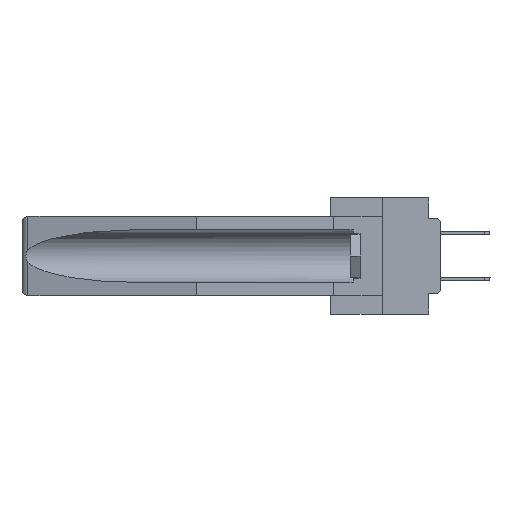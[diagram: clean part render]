
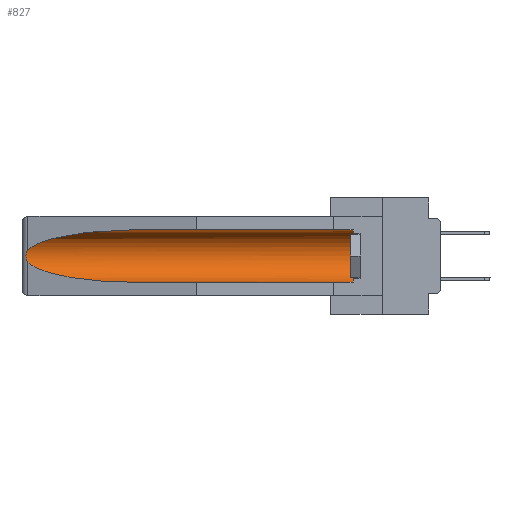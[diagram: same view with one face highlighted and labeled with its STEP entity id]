
A CAD part, left-side view. The second image highlights one B-rep face of the part: STEP entity #827.
In plain terms, the highlighted cylindrical face has radius 2.857 mm (diameter 5.715 mm), a partial arc.
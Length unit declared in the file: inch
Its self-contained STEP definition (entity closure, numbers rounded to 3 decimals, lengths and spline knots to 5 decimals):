
#441 = CARTESIAN_POINT ( 'NONE',  ( 0.2673, 1.5327, -0.16383 ) ) ;
#774 = CIRCLE ( 'NONE', #2671, 0.1125 ) ;
#827 = ADVANCED_FACE ( 'NONE', ( #22563 ), #9307, .F. ) ;
#1045 = CARTESIAN_POINT ( 'NONE',  ( 0.155, 1.07973, -0.059 ) ) ;
#1121 = CARTESIAN_POINT ( 'NONE',  ( 0.155, 1.07973, -0.284 ) ) ;
#1220 = CARTESIAN_POINT ( 'NONE',  ( 0.155, 1.07973, -0.059 ) ) ;
#1238 = ORIENTED_EDGE ( 'NONE', *, *, #25741, .T. ) ;
#1357 = CARTESIAN_POINT ( 'NONE',  ( 0.155, 0.126, -0.284 ) ) ;
#1448 = CARTESIAN_POINT ( 'NONE',  ( 0.26537, 1.52718, -0.14972 ) ) ;
#1894 = AXIS2_PLACEMENT_3D ( 'NONE', #6697, #4351, #22425 ) ;
#2671 = AXIS2_PLACEMENT_3D ( 'NONE', #27612, #11398, #7012 ) ;
#2932 = CARTESIAN_POINT ( 'NONE',  ( 0.2673, 1.53269, -0.17917 ) ) ;
#3207 = VERTEX_POINT ( 'NONE', #1121 ) ;
#4351 = DIRECTION ( 'NONE',  ( 0., 1., 0. ) ) ;
#5395 = CARTESIAN_POINT ( 'NONE',  ( 0.155, -0.30754, -0.059 ) ) ;
#6697 = CARTESIAN_POINT ( 'NONE',  ( 0.155, -0.30754, -0.1715 ) ) ;
#7012 = DIRECTION ( 'NONE',  ( 0., 0., 1. ) ) ;
#7700 = CARTESIAN_POINT ( 'NONE',  ( 0.25451, 1.48313, -0.24835 ) ) ;
#7730 = VERTEX_POINT ( 'NONE', #1357 ) ;
#8001 = CARTESIAN_POINT ( 'NONE',  ( 0.21114, 1.30732, -0.284 ) ) ;
#9307 = CYLINDRICAL_SURFACE ( 'NONE', #1894, 0.1125 ) ;
#9392 = CARTESIAN_POINT ( 'NONE',  ( 0.26597, 1.52961, -0.15275 ) ) ;
#10302 = CARTESIAN_POINT ( 'NONE',  ( 0.25451, 1.48313, -0.09465 ) ) ;
#11138 = VECTOR ( 'NONE', #12366, 39.37008 ) ;
#11343 = ORIENTED_EDGE ( 'NONE', *, *, #18758, .T. ) ;
#11398 = DIRECTION ( 'NONE',  ( 0., -1., 0. ) ) ;
#11415 = VERTEX_POINT ( 'NONE', #1448 ) ;
#11786 = CARTESIAN_POINT ( 'NONE',  ( 0.155, 0.126, -0.059 ) ) ;
#11888 = CARTESIAN_POINT ( 'NONE',  ( 0.26537, 1.52718, -0.19328 ) ) ;
#12366 = DIRECTION ( 'NONE',  ( 0., 1., 0. ) ) ;
#14098 = CARTESIAN_POINT ( 'NONE',  ( 0.26654, 1.53092, -0.15636 ) ) ;
#14947 = VECTOR ( 'NONE', #24578, 39.37008 ) ;
#15572 = ORIENTED_EDGE ( 'NONE', *, *, #17820, .T. ) ;
#16286 = CARTESIAN_POINT ( 'NONE',  ( 0.26537, 1.52718, -0.14972 ) ) ;
#16301 = ORIENTED_EDGE ( 'NONE', *, *, #27776, .T. ) ;
#16391 = EDGE_LOOP ( 'NONE', ( #11343, #16301, #1238, #21153, #17786, #15572 ) ) ;
#16468 = EDGE_CURVE ( 'NONE', #7730, #21875, #774, .T. ) ;
#16647 = CARTESIAN_POINT ( 'NONE',  ( 0.155, 1.07973, -0.284 ) ) ;
#17065 = CARTESIAN_POINT ( 'NONE',  ( 0.26537, 1.52718, -0.14972 ) ) ;
#17400 = EDGE_CURVE ( 'NONE', #7730, #3207, #20894, .T. ) ;
#17786 = ORIENTED_EDGE ( 'NONE', *, *, #16468, .T. ) ;
#17820 = EDGE_CURVE ( 'NONE', #21875, #26985, #26948, .T. ) ;
#18070 = CARTESIAN_POINT ( 'NONE',  ( 0.2675, 1.53308, -0.16763 ) ) ;
#18363 = CARTESIAN_POINT ( 'NONE',  ( 0.2675, 1.53308, -0.17534 ) ) ;
#18758 = EDGE_CURVE ( 'NONE', #26985, #11415, #19409, .T. ) ;
#19409 =( BOUNDED_CURVE ( )  B_SPLINE_CURVE ( 3, ( #1045, #21054, #10302, #17065 ),
 .UNSPECIFIED., .F., .F. ) 
 B_SPLINE_CURVE_WITH_KNOTS ( ( 4, 4 ),
 ( 4.71239, 6.08839 ),
 .UNSPECIFIED. ) 
 CURVE ( )  GEOMETRIC_REPRESENTATION_ITEM ( )  RATIONAL_B_SPLINE_CURVE ( ( 1., 0.848, 0.848, 1. ) ) 
 REPRESENTATION_ITEM ( '' )  );
#19684 = CARTESIAN_POINT ( 'NONE',  ( 0.26537, 1.52718, -0.19328 ) ) ;
#20894 = LINE ( 'NONE', #21046, #11138 ) ;
#21046 = CARTESIAN_POINT ( 'NONE',  ( 0.155, -0.30754, -0.284 ) ) ;
#21054 = CARTESIAN_POINT ( 'NONE',  ( 0.21114, 1.30732, -0.059 ) ) ;
#21153 = ORIENTED_EDGE ( 'NONE', *, *, #17400, .F. ) ;
#21875 = VERTEX_POINT ( 'NONE', #11786 ) ;
#22425 = DIRECTION ( 'NONE',  ( 0., 0., 1. ) ) ;
#22563 = FACE_OUTER_BOUND ( 'NONE', #16391, .T. ) ;
#22643 = CARTESIAN_POINT ( 'NONE',  ( 0.26597, 1.5296, -0.19026 ) ) ;
#24168 =( BOUNDED_CURVE ( )  B_SPLINE_CURVE ( 3, ( #28175, #7700, #8001, #16647 ),
 .UNSPECIFIED., .F., .F. ) 
 B_SPLINE_CURVE_WITH_KNOTS ( ( 4, 4 ),
 ( 0.1948, 1.5708 ),
 .UNSPECIFIED. ) 
 CURVE ( )  GEOMETRIC_REPRESENTATION_ITEM ( )  RATIONAL_B_SPLINE_CURVE ( ( 1., 0.848, 0.848, 1. ) ) 
 REPRESENTATION_ITEM ( '' )  );
#24578 = DIRECTION ( 'NONE',  ( 0., 1., 0. ) ) ;
#25022 = B_SPLINE_CURVE_WITH_KNOTS ( 'NONE', 3,
 ( #16286, #9392, #14098, #441, #18070, #18363, #2932, #27367, #22643, #11888 ),
 .UNSPECIFIED., .F., .F.,
 ( 4, 2, 2, 2, 4 ),
 ( 0., 0.00029, 0.00058, 0.00087, 0.00117 ),
 .UNSPECIFIED. ) ;
#25741 = EDGE_CURVE ( 'NONE', #28022, #3207, #24168, .T. ) ;
#26948 = LINE ( 'NONE', #5395, #14947 ) ;
#26985 = VERTEX_POINT ( 'NONE', #1220 ) ;
#27367 = CARTESIAN_POINT ( 'NONE',  ( 0.26655, 1.53094, -0.18657 ) ) ;
#27612 = CARTESIAN_POINT ( 'NONE',  ( 0.155, 0.126, -0.1715 ) ) ;
#27776 = EDGE_CURVE ( 'NONE', #11415, #28022, #25022, .T. ) ;
#28022 = VERTEX_POINT ( 'NONE', #19684 ) ;
#28175 = CARTESIAN_POINT ( 'NONE',  ( 0.26537, 1.52718, -0.19328 ) ) ;
